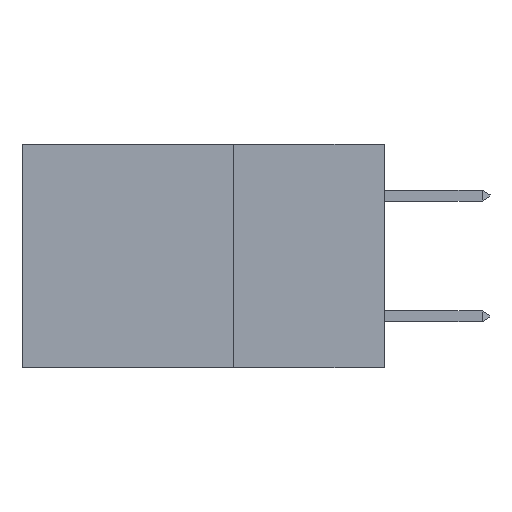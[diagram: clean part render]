
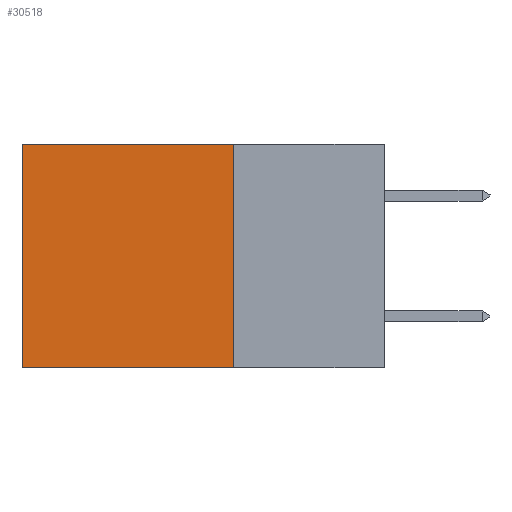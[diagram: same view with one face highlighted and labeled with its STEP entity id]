
A CAD part, left-side view. The second image highlights one B-rep face of the part: STEP entity #30518.
In plain terms, the highlighted planar face has unit normal (-1, 0, 0).
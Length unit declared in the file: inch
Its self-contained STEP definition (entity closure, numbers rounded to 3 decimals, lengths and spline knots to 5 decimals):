
#2083 = CARTESIAN_POINT ( 'NONE',  ( 0.2875, 0.25, 0. ) ) ;
#2549 = ORIENTED_EDGE ( 'NONE', *, *, #24805, .F. ) ;
#4929 = LINE ( 'NONE', #11575, #31355 ) ;
#9209 = EDGE_CURVE ( 'NONE', #25702, #27864, #25010, .T. ) ;
#10883 = LINE ( 'NONE', #16568, #33005 ) ;
#10954 = FACE_OUTER_BOUND ( 'NONE', #18817, .T. ) ;
#11575 = CARTESIAN_POINT ( 'NONE',  ( 0.2875, 0.6, 0. ) ) ;
#11746 = CARTESIAN_POINT ( 'NONE',  ( 0.2875, 0.25, 0. ) ) ;
#12027 = DIRECTION ( 'NONE',  ( 0., 0., -1. ) ) ;
#12599 = PLANE ( 'NONE',  #28073 ) ;
#12933 = DIRECTION ( 'NONE',  ( 0., 1., 0. ) ) ;
#13797 = ORIENTED_EDGE ( 'NONE', *, *, #9209, .F. ) ;
#16568 = CARTESIAN_POINT ( 'NONE',  ( 0.2875, 0.25, 0. ) ) ;
#18298 = CARTESIAN_POINT ( 'NONE',  ( 0.2875, 0.25, -0.37 ) ) ;
#18817 = EDGE_LOOP ( 'NONE', ( #40980, #13797, #2549, #39387 ) ) ;
#23940 = VECTOR ( 'NONE', #12933, 39.37008 ) ;
#24549 = EDGE_CURVE ( 'NONE', #35107, #27864, #4929, .T. ) ;
#24792 = EDGE_CURVE ( 'NONE', #29903, #35107, #10883, .T. ) ;
#24805 = EDGE_CURVE ( 'NONE', #29903, #25702, #37340, .T. ) ;
#25010 = LINE ( 'NONE', #37435, #23940 ) ;
#25702 = VERTEX_POINT ( 'NONE', #18298 ) ;
#27864 = VERTEX_POINT ( 'NONE', #37456 ) ;
#28073 = AXIS2_PLACEMENT_3D ( 'NONE', #2083, #40232, #29336 ) ;
#29336 = DIRECTION ( 'NONE',  ( 0., 0., -1. ) ) ;
#29903 = VERTEX_POINT ( 'NONE', #11746 ) ;
#30449 = CARTESIAN_POINT ( 'NONE',  ( 0.2875, 0.6, 0. ) ) ;
#30518 = ADVANCED_FACE ( 'NONE', ( #10954 ), #12599, .F. ) ;
#31355 = VECTOR ( 'NONE', #12027, 39.37008 ) ;
#33005 = VECTOR ( 'NONE', #41141, 39.37008 ) ;
#35107 = VERTEX_POINT ( 'NONE', #30449 ) ;
#37340 = LINE ( 'NONE', #44203, #44338 ) ;
#37435 = CARTESIAN_POINT ( 'NONE',  ( 0.2875, 0.25, -0.37 ) ) ;
#37456 = CARTESIAN_POINT ( 'NONE',  ( 0.2875, 0.6, -0.37 ) ) ;
#37711 = DIRECTION ( 'NONE',  ( 0., 0., -1. ) ) ;
#39387 = ORIENTED_EDGE ( 'NONE', *, *, #24792, .T. ) ;
#40232 = DIRECTION ( 'NONE',  ( 1., 0., 0. ) ) ;
#40980 = ORIENTED_EDGE ( 'NONE', *, *, #24549, .T. ) ;
#41141 = DIRECTION ( 'NONE',  ( 0., 1., 0. ) ) ;
#44203 = CARTESIAN_POINT ( 'NONE',  ( 0.2875, 0.25, 0. ) ) ;
#44338 = VECTOR ( 'NONE', #37711, 39.37008 ) ;
